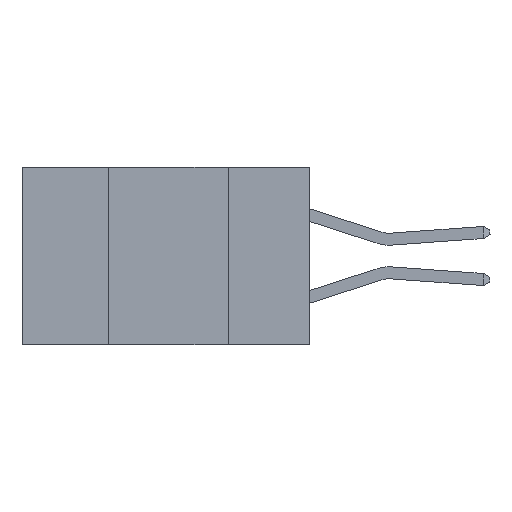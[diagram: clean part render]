
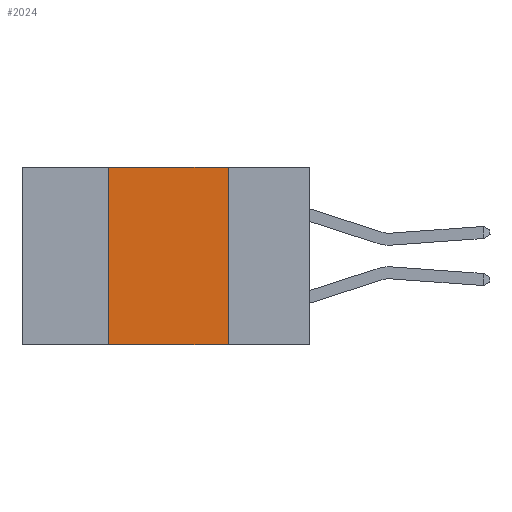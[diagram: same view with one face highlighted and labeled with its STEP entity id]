
A CAD part, left-side view. The second image highlights one B-rep face of the part: STEP entity #2024.
In plain terms, the highlighted planar face has unit normal (-1, 0, 0).
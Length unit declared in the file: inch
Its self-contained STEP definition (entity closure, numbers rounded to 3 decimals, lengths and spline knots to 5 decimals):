
#238 = EDGE_LOOP ( 'NONE', ( #2888, #7014, #8764, #2750 ) ) ;
#349 = EDGE_CURVE ( 'NONE', #11462, #6029, #9469, .T. ) ;
#496 = AXIS2_PLACEMENT_3D ( 'NONE', #11047, #11596, #11566 ) ;
#922 = VECTOR ( 'NONE', #12454, 39.37008 ) ;
#1307 = CARTESIAN_POINT ( 'NONE',  ( 0., 0.6, -0.37 ) ) ;
#2024 = ADVANCED_FACE ( 'NONE', ( #3033 ), #11093, .F. ) ;
#2750 = ORIENTED_EDGE ( 'NONE', *, *, #13193, .T. ) ;
#2888 = ORIENTED_EDGE ( 'NONE', *, *, #14002, .F. ) ;
#3033 = FACE_OUTER_BOUND ( 'NONE', #238, .T. ) ;
#3664 = LINE ( 'NONE', #1307, #12279 ) ;
#4877 = CARTESIAN_POINT ( 'NONE',  ( 0., 0.17, -0.37 ) ) ;
#5032 = VERTEX_POINT ( 'NONE', #7829 ) ;
#6029 = VERTEX_POINT ( 'NONE', #14063 ) ;
#7014 = ORIENTED_EDGE ( 'NONE', *, *, #349, .F. ) ;
#7829 = CARTESIAN_POINT ( 'NONE',  ( 0., 0.42, -0.37 ) ) ;
#7897 = VECTOR ( 'NONE', #9707, 39.37008 ) ;
#8764 = ORIENTED_EDGE ( 'NONE', *, *, #9817, .F. ) ;
#9178 = VERTEX_POINT ( 'NONE', #4877 ) ;
#9301 = DIRECTION ( 'NONE',  ( 0., -1., 0. ) ) ;
#9469 = LINE ( 'NONE', #9954, #12048 ) ;
#9487 = CARTESIAN_POINT ( 'NONE',  ( 0., 0.42, 0. ) ) ;
#9686 = LINE ( 'NONE', #11385, #922 ) ;
#9707 = DIRECTION ( 'NONE',  ( 0., 0., 1. ) ) ;
#9791 = CARTESIAN_POINT ( 'NONE',  ( 0., 0.42, -0.37 ) ) ;
#9817 = EDGE_CURVE ( 'NONE', #5032, #11462, #10875, .T. ) ;
#9954 = CARTESIAN_POINT ( 'NONE',  ( 0., 0.6, 0. ) ) ;
#10875 = LINE ( 'NONE', #9791, #7897 ) ;
#11047 = CARTESIAN_POINT ( 'NONE',  ( 0., 0.6, 0. ) ) ;
#11093 = PLANE ( 'NONE',  #496 ) ;
#11385 = CARTESIAN_POINT ( 'NONE',  ( 0., 0.17, -0.37 ) ) ;
#11462 = VERTEX_POINT ( 'NONE', #9487 ) ;
#11566 = DIRECTION ( 'NONE',  ( 0., 0., -1. ) ) ;
#11596 = DIRECTION ( 'NONE',  ( 1., 0., 0. ) ) ;
#12048 = VECTOR ( 'NONE', #14562, 39.37008 ) ;
#12279 = VECTOR ( 'NONE', #9301, 39.37008 ) ;
#12454 = DIRECTION ( 'NONE',  ( 0., 0., -1. ) ) ;
#13193 = EDGE_CURVE ( 'NONE', #5032, #9178, #3664, .T. ) ;
#14002 = EDGE_CURVE ( 'NONE', #6029, #9178, #9686, .T. ) ;
#14063 = CARTESIAN_POINT ( 'NONE',  ( 0., 0.17, 0. ) ) ;
#14562 = DIRECTION ( 'NONE',  ( 0., -1., 0. ) ) ;
